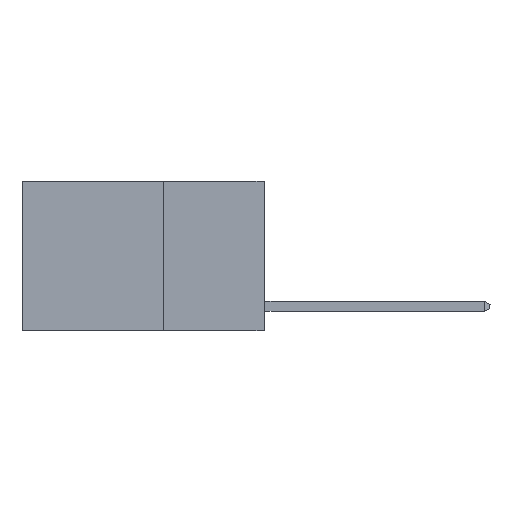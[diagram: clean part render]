
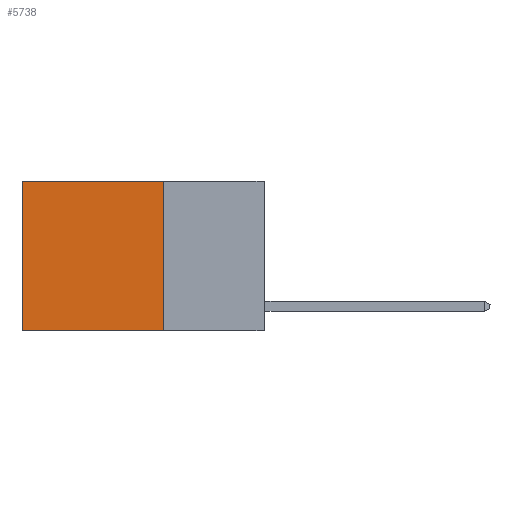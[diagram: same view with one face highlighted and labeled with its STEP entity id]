
A CAD part, left-side view. The second image highlights one B-rep face of the part: STEP entity #5738.
In plain terms, the highlighted planar face has unit normal (-1, 0, 0).
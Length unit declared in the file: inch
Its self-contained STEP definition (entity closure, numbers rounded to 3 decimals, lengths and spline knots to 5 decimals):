
#144 = VERTEX_POINT ( 'NONE', #11073 ) ;
#220 = LINE ( 'NONE', #561, #3672 ) ;
#414 = EDGE_CURVE ( 'NONE', #2946, #144, #10349, .T. ) ;
#561 = CARTESIAN_POINT ( 'NONE',  ( 0.2625, 0.25, 0. ) ) ;
#824 = PLANE ( 'NONE',  #10801 ) ;
#1239 = VERTEX_POINT ( 'NONE', #4498 ) ;
#1805 = ORIENTED_EDGE ( 'NONE', *, *, #414, .T. ) ;
#2759 = DIRECTION ( 'NONE',  ( 0., 0., -1. ) ) ;
#2841 = LINE ( 'NONE', #7994, #5909 ) ;
#2946 = VERTEX_POINT ( 'NONE', #6887 ) ;
#3521 = LINE ( 'NONE', #7742, #8687 ) ;
#3661 = FACE_OUTER_BOUND ( 'NONE', #10858, .T. ) ;
#3672 = VECTOR ( 'NONE', #4003, 39.37008 ) ;
#4003 = DIRECTION ( 'NONE',  ( 0., 0., -1. ) ) ;
#4324 = VECTOR ( 'NONE', #11258, 39.37008 ) ;
#4498 = CARTESIAN_POINT ( 'NONE',  ( 0.2625, 0.6, -0.37 ) ) ;
#4543 = CARTESIAN_POINT ( 'NONE',  ( 0.2625, 0.25, 0. ) ) ;
#4989 = EDGE_CURVE ( 'NONE', #9199, #1239, #3521, .T. ) ;
#5179 = DIRECTION ( 'NONE',  ( 0., 1., 0. ) ) ;
#5329 = DIRECTION ( 'NONE',  ( 0., 0., -1. ) ) ;
#5738 = ADVANCED_FACE ( 'NONE', ( #3661 ), #824, .F. ) ;
#5863 = CARTESIAN_POINT ( 'NONE',  ( 0.2625, 0.25, 0. ) ) ;
#5909 = VECTOR ( 'NONE', #5329, 39.37008 ) ;
#6473 = ORIENTED_EDGE ( 'NONE', *, *, #7616, .F. ) ;
#6758 = ORIENTED_EDGE ( 'NONE', *, *, #7350, .T. ) ;
#6887 = CARTESIAN_POINT ( 'NONE',  ( 0.2625, 0.25, 0. ) ) ;
#7074 = ORIENTED_EDGE ( 'NONE', *, *, #4989, .F. ) ;
#7350 = EDGE_CURVE ( 'NONE', #144, #1239, #2841, .T. ) ;
#7616 = EDGE_CURVE ( 'NONE', #2946, #9199, #220, .T. ) ;
#7742 = CARTESIAN_POINT ( 'NONE',  ( 0.2625, 0.25, -0.37 ) ) ;
#7994 = CARTESIAN_POINT ( 'NONE',  ( 0.2625, 0.6, 0. ) ) ;
#8687 = VECTOR ( 'NONE', #5179, 39.37008 ) ;
#9199 = VERTEX_POINT ( 'NONE', #9955 ) ;
#9955 = CARTESIAN_POINT ( 'NONE',  ( 0.2625, 0.25, -0.37 ) ) ;
#10349 = LINE ( 'NONE', #5863, #4324 ) ;
#10676 = DIRECTION ( 'NONE',  ( 1., 0., 0. ) ) ;
#10801 = AXIS2_PLACEMENT_3D ( 'NONE', #4543, #10676, #2759 ) ;
#10858 = EDGE_LOOP ( 'NONE', ( #6758, #7074, #6473, #1805 ) ) ;
#11073 = CARTESIAN_POINT ( 'NONE',  ( 0.2625, 0.6, 0. ) ) ;
#11258 = DIRECTION ( 'NONE',  ( 0., 1., 0. ) ) ;
